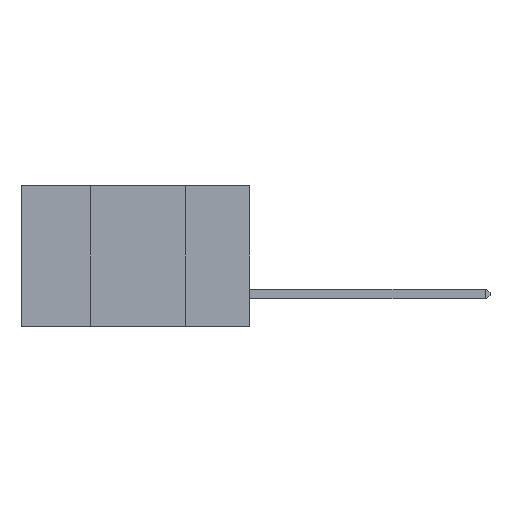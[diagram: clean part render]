
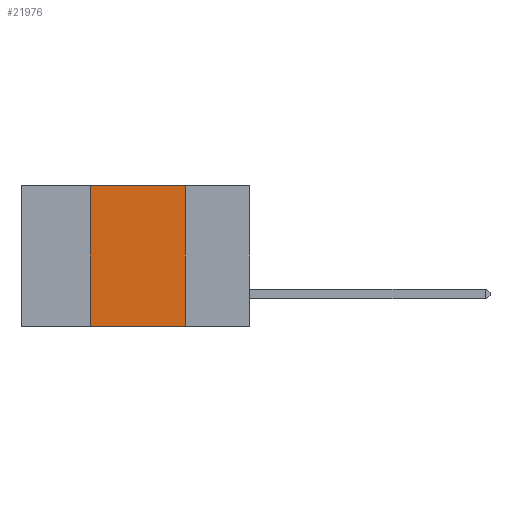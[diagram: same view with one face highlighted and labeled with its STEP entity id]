
A CAD part, left-side view. The second image highlights one B-rep face of the part: STEP entity #21976.
In plain terms, the highlighted planar face has unit normal (-1, 0, 0).
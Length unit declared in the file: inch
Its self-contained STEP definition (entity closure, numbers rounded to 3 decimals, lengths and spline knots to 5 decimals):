
#1980 = EDGE_CURVE ( 'NONE', #7683, #3934, #31899, .T. ) ;
#2756 = VECTOR ( 'NONE', #22396, 39.37008 ) ;
#3613 = LINE ( 'NONE', #27800, #2756 ) ;
#3934 = VERTEX_POINT ( 'NONE', #19892 ) ;
#5042 = ORIENTED_EDGE ( 'NONE', *, *, #16887, .T. ) ;
#7683 = VERTEX_POINT ( 'NONE', #24413 ) ;
#8047 = VECTOR ( 'NONE', #32136, 39.37008 ) ;
#9271 = VECTOR ( 'NONE', #9572, 39.37008 ) ;
#9572 = DIRECTION ( 'NONE',  ( 0., 0., -1. ) ) ;
#9746 = LINE ( 'NONE', #29465, #8047 ) ;
#10337 = CARTESIAN_POINT ( 'NONE',  ( 0., 0.6, 0. ) ) ;
#10440 = DIRECTION ( 'NONE',  ( 1., 0., 0. ) ) ;
#11429 = AXIS2_PLACEMENT_3D ( 'NONE', #10337, #10440, #29622 ) ;
#12537 = VERTEX_POINT ( 'NONE', #12679 ) ;
#12679 = CARTESIAN_POINT ( 'NONE',  ( 0., 0.42, -0.37 ) ) ;
#13388 = EDGE_CURVE ( 'NONE', #12537, #23816, #3613, .T. ) ;
#14100 = EDGE_LOOP ( 'NONE', ( #20897, #31101, #31276, #5042 ) ) ;
#14894 = CARTESIAN_POINT ( 'NONE',  ( 0., 0.6, -0.37 ) ) ;
#15512 = DIRECTION ( 'NONE',  ( 0., -1., 0. ) ) ;
#15834 = PLANE ( 'NONE',  #11429 ) ;
#16887 = EDGE_CURVE ( 'NONE', #12537, #3934, #30357, .T. ) ;
#18013 = CARTESIAN_POINT ( 'NONE',  ( 0., 0.42, 0. ) ) ;
#18796 = EDGE_CURVE ( 'NONE', #23816, #7683, #9746, .T. ) ;
#19892 = CARTESIAN_POINT ( 'NONE',  ( 0., 0.17, -0.37 ) ) ;
#20489 = CARTESIAN_POINT ( 'NONE',  ( 0., 0.17, 0. ) ) ;
#20897 = ORIENTED_EDGE ( 'NONE', *, *, #1980, .F. ) ;
#21976 = ADVANCED_FACE ( 'NONE', ( #25022 ), #15834, .F. ) ;
#22396 = DIRECTION ( 'NONE',  ( 0., 0., 1. ) ) ;
#23126 = VECTOR ( 'NONE', #15512, 39.37008 ) ;
#23816 = VERTEX_POINT ( 'NONE', #18013 ) ;
#24413 = CARTESIAN_POINT ( 'NONE',  ( 0., 0.17, 0. ) ) ;
#25022 = FACE_OUTER_BOUND ( 'NONE', #14100, .T. ) ;
#27800 = CARTESIAN_POINT ( 'NONE',  ( 0., 0.42, 0. ) ) ;
#29465 = CARTESIAN_POINT ( 'NONE',  ( 0., 0.6, 0. ) ) ;
#29622 = DIRECTION ( 'NONE',  ( 0., 0., -1. ) ) ;
#30357 = LINE ( 'NONE', #14894, #23126 ) ;
#31101 = ORIENTED_EDGE ( 'NONE', *, *, #18796, .F. ) ;
#31276 = ORIENTED_EDGE ( 'NONE', *, *, #13388, .F. ) ;
#31899 = LINE ( 'NONE', #20489, #9271 ) ;
#32136 = DIRECTION ( 'NONE',  ( 0., -1., 0. ) ) ;
